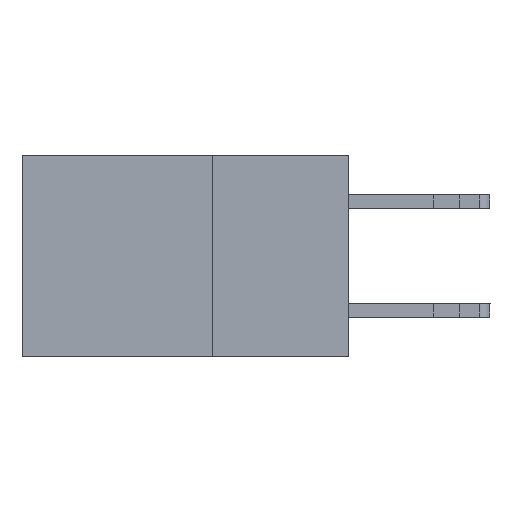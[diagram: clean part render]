
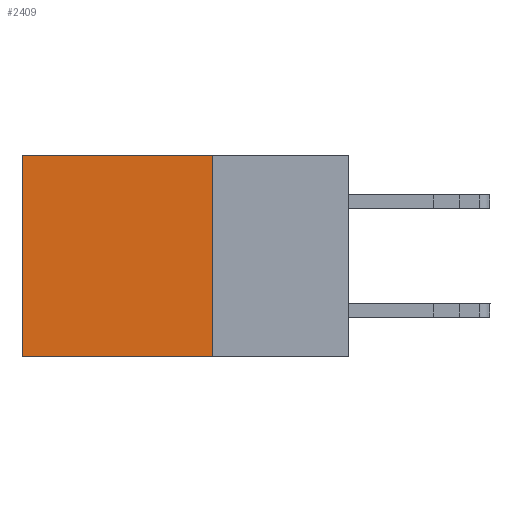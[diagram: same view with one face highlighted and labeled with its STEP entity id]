
A CAD part, left-side view. The second image highlights one B-rep face of the part: STEP entity #2409.
In plain terms, the highlighted planar face has unit normal (-1, 0, 0).
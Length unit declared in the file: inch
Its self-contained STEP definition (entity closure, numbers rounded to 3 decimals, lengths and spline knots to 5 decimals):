
#838 = ORIENTED_EDGE ( 'NONE', *, *, #11603, .T. ) ;
#1469 = VECTOR ( 'NONE', #5106, 39.37008 ) ;
#2055 = VECTOR ( 'NONE', #6935, 39.37008 ) ;
#2156 = DIRECTION ( 'NONE',  ( 0., 0., -1. ) ) ;
#2409 = ADVANCED_FACE ( 'NONE', ( #3290 ), #6648, .F. ) ;
#2412 = CARTESIAN_POINT ( 'NONE',  ( 0.298, 0.25, 0. ) ) ;
#2565 = CARTESIAN_POINT ( 'NONE',  ( 0.298, 0.25, 0. ) ) ;
#2823 = AXIS2_PLACEMENT_3D ( 'NONE', #2565, #5653, #5532 ) ;
#2870 = VERTEX_POINT ( 'NONE', #2412 ) ;
#3096 = VERTEX_POINT ( 'NONE', #10849 ) ;
#3202 = ORIENTED_EDGE ( 'NONE', *, *, #7611, .T. ) ;
#3290 = FACE_OUTER_BOUND ( 'NONE', #5753, .T. ) ;
#3296 = DIRECTION ( 'NONE',  ( 0., 1., 0. ) ) ;
#3306 = CARTESIAN_POINT ( 'NONE',  ( 0.298, 0.6, -0.37 ) ) ;
#4888 = ORIENTED_EDGE ( 'NONE', *, *, #11651, .F. ) ;
#5032 = CARTESIAN_POINT ( 'NONE',  ( 0.298, 0.25, 0. ) ) ;
#5071 = VECTOR ( 'NONE', #3296, 39.37008 ) ;
#5106 = DIRECTION ( 'NONE',  ( 0., 1., 0. ) ) ;
#5532 = DIRECTION ( 'NONE',  ( 0., 0., -1. ) ) ;
#5653 = DIRECTION ( 'NONE',  ( 1., 0., 0. ) ) ;
#5753 = EDGE_LOOP ( 'NONE', ( #838, #11921, #4888, #3202 ) ) ;
#6057 = CARTESIAN_POINT ( 'NONE',  ( 0.298, 0.25, -0.37 ) ) ;
#6527 = EDGE_CURVE ( 'NONE', #11967, #6710, #10838, .T. ) ;
#6648 = PLANE ( 'NONE',  #2823 ) ;
#6710 = VERTEX_POINT ( 'NONE', #3306 ) ;
#6935 = DIRECTION ( 'NONE',  ( 0., 0., -1. ) ) ;
#7611 = EDGE_CURVE ( 'NONE', #2870, #3096, #9518, .T. ) ;
#7751 = VECTOR ( 'NONE', #2156, 39.37008 ) ;
#9518 = LINE ( 'NONE', #11293, #5071 ) ;
#10157 = LINE ( 'NONE', #5032, #7751 ) ;
#10813 = LINE ( 'NONE', #12915, #2055 ) ;
#10838 = LINE ( 'NONE', #6057, #1469 ) ;
#10849 = CARTESIAN_POINT ( 'NONE',  ( 0.298, 0.6, 0. ) ) ;
#11293 = CARTESIAN_POINT ( 'NONE',  ( 0.298, 0.25, 0. ) ) ;
#11603 = EDGE_CURVE ( 'NONE', #3096, #6710, #10813, .T. ) ;
#11651 = EDGE_CURVE ( 'NONE', #2870, #11967, #10157, .T. ) ;
#11921 = ORIENTED_EDGE ( 'NONE', *, *, #6527, .F. ) ;
#11967 = VERTEX_POINT ( 'NONE', #12618 ) ;
#12618 = CARTESIAN_POINT ( 'NONE',  ( 0.298, 0.25, -0.37 ) ) ;
#12915 = CARTESIAN_POINT ( 'NONE',  ( 0.298, 0.6, 0. ) ) ;
